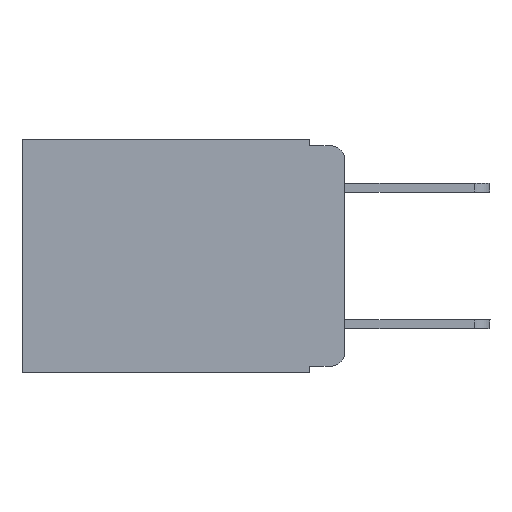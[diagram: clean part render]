
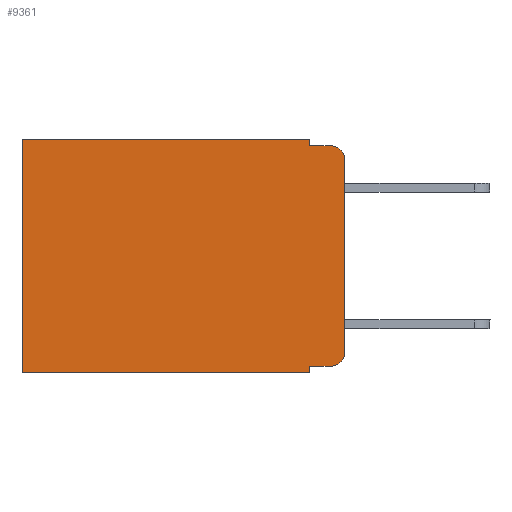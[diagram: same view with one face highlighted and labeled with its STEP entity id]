
A CAD part, left-side view. The second image highlights one B-rep face of the part: STEP entity #9361.
In plain terms, the highlighted planar face has unit normal (-1, 0, 0).
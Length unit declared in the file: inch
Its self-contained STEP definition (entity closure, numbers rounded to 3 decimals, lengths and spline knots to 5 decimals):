
#227 = EDGE_CURVE ( 'NONE', #283, #7576, #11471, .T. ) ;
#258 = VERTEX_POINT ( 'NONE', #7522 ) ;
#283 = VERTEX_POINT ( 'NONE', #7147 ) ;
#375 = CARTESIAN_POINT ( 'NONE',  ( 0.298, 0.051, -0.333 ) ) ;
#421 = EDGE_CURVE ( 'NONE', #11881, #6773, #3278, .T. ) ;
#482 = LINE ( 'NONE', #7294, #11235 ) ;
#676 = VECTOR ( 'NONE', #5127, 39.37008 ) ;
#820 = CARTESIAN_POINT ( 'NONE',  ( 0.298, 0., -0.03 ) ) ;
#1162 = CARTESIAN_POINT ( 'NONE',  ( 0.298, 0., 0. ) ) ;
#1236 = ORIENTED_EDGE ( 'NONE', *, *, #6168, .F. ) ;
#1543 = EDGE_CURVE ( 'NONE', #7630, #258, #12568, .T. ) ;
#1599 = DIRECTION ( 'NONE',  ( -1., 0., 0. ) ) ;
#1777 = CARTESIAN_POINT ( 'NONE',  ( 0.298, 0.051, 0. ) ) ;
#1807 = DIRECTION ( 'NONE',  ( -1., 0., 0. ) ) ;
#2048 = CARTESIAN_POINT ( 'NONE',  ( 0.298, 0.051, 0. ) ) ;
#2175 = FACE_OUTER_BOUND ( 'NONE', #10847, .T. ) ;
#2257 = ORIENTED_EDGE ( 'NONE', *, *, #9995, .T. ) ;
#2835 = CARTESIAN_POINT ( 'NONE',  ( 0.298, 0.473, 0. ) ) ;
#3069 = ORIENTED_EDGE ( 'NONE', *, *, #421, .T. ) ;
#3278 = LINE ( 'NONE', #2835, #5050 ) ;
#3496 = DIRECTION ( 'NONE',  ( 0., -1., 0. ) ) ;
#3521 = CARTESIAN_POINT ( 'NONE',  ( 0.298, 0., 0. ) ) ;
#3684 = DIRECTION ( 'NONE',  ( 0., 0., -1. ) ) ;
#3788 = ORIENTED_EDGE ( 'NONE', *, *, #8992, .T. ) ;
#4166 = AXIS2_PLACEMENT_3D ( 'NONE', #6722, #1599, #8792 ) ;
#4220 = ORIENTED_EDGE ( 'NONE', *, *, #9329, .T. ) ;
#4440 = VERTEX_POINT ( 'NONE', #13296 ) ;
#4481 = CIRCLE ( 'NONE', #7129, 0.02 ) ;
#4566 = CARTESIAN_POINT ( 'NONE',  ( 0.298, 0.051, -0.333 ) ) ;
#4683 = CARTESIAN_POINT ( 'NONE',  ( 0.298, 0.051, 0. ) ) ;
#4731 = DIRECTION ( 'NONE',  ( 0., 0., -1. ) ) ;
#5050 = VECTOR ( 'NONE', #8057, 39.37008 ) ;
#5127 = DIRECTION ( 'NONE',  ( 0., -1., 0. ) ) ;
#5599 = VECTOR ( 'NONE', #5652, 39.37008 ) ;
#5652 = DIRECTION ( 'NONE',  ( 0., 1., 0. ) ) ;
#5732 = EDGE_CURVE ( 'NONE', #7428, #11795, #11830, .T. ) ;
#6144 = VECTOR ( 'NONE', #3496, 39.37008 ) ;
#6168 = EDGE_CURVE ( 'NONE', #4440, #6773, #482, .T. ) ;
#6326 = DIRECTION ( 'NONE',  ( 0., 1., 0. ) ) ;
#6331 = DIRECTION ( 'NONE',  ( 0., 0., -1. ) ) ;
#6357 = EDGE_CURVE ( 'NONE', #8058, #283, #6925, .T. ) ;
#6407 = ORIENTED_EDGE ( 'NONE', *, *, #1543, .T. ) ;
#6462 = VECTOR ( 'NONE', #4731, 39.37008 ) ;
#6722 = CARTESIAN_POINT ( 'NONE',  ( 0.298, 0.02, -0.313 ) ) ;
#6773 = VERTEX_POINT ( 'NONE', #9364 ) ;
#6925 = LINE ( 'NONE', #4683, #8186 ) ;
#7129 = AXIS2_PLACEMENT_3D ( 'NONE', #11010, #1807, #12092 ) ;
#7147 = CARTESIAN_POINT ( 'NONE',  ( 0.298, 0.051, -0.01 ) ) ;
#7247 = LINE ( 'NONE', #1777, #6462 ) ;
#7294 = CARTESIAN_POINT ( 'NONE',  ( 0.298, 0., -0.343 ) ) ;
#7428 = VERTEX_POINT ( 'NONE', #820 ) ;
#7522 = CARTESIAN_POINT ( 'NONE',  ( 0.298, 0.02, -0.333 ) ) ;
#7576 = VERTEX_POINT ( 'NONE', #12349 ) ;
#7630 = VERTEX_POINT ( 'NONE', #4566 ) ;
#7655 = LINE ( 'NONE', #1162, #5599 ) ;
#8057 = DIRECTION ( 'NONE',  ( 0., 0., -1. ) ) ;
#8058 = VERTEX_POINT ( 'NONE', #2048 ) ;
#8186 = VECTOR ( 'NONE', #3684, 39.37008 ) ;
#8372 = ORIENTED_EDGE ( 'NONE', *, *, #6357, .F. ) ;
#8576 = CARTESIAN_POINT ( 'NONE',  ( 0.298, 0.473, 0. ) ) ;
#8736 = DIRECTION ( 'NONE',  ( 0., 0., -1. ) ) ;
#8792 = DIRECTION ( 'NONE',  ( 0., 0., -1. ) ) ;
#8872 = AXIS2_PLACEMENT_3D ( 'NONE', #3521, #11701, #8736 ) ;
#8992 = EDGE_CURVE ( 'NONE', #7428, #7576, #4481, .T. ) ;
#9329 = EDGE_CURVE ( 'NONE', #8058, #11881, #7655, .T. ) ;
#9361 = ADVANCED_FACE ( 'NONE', ( #2175 ), #9617, .F. ) ;
#9364 = CARTESIAN_POINT ( 'NONE',  ( 0.298, 0.473, -0.343 ) ) ;
#9617 = PLANE ( 'NONE',  #8872 ) ;
#9708 = ORIENTED_EDGE ( 'NONE', *, *, #227, .F. ) ;
#9995 = EDGE_CURVE ( 'NONE', #258, #11795, #12284, .T. ) ;
#10327 = CARTESIAN_POINT ( 'NONE',  ( 0.298, 0., 0. ) ) ;
#10734 = CARTESIAN_POINT ( 'NONE',  ( 0.298, 0., -0.313 ) ) ;
#10847 = EDGE_LOOP ( 'NONE', ( #11048, #3788, #9708, #8372, #4220, #3069, #1236, #10872, #6407, #2257 ) ) ;
#10872 = ORIENTED_EDGE ( 'NONE', *, *, #12462, .F. ) ;
#10904 = CARTESIAN_POINT ( 'NONE',  ( 0.298, 0.051, -0.01 ) ) ;
#11010 = CARTESIAN_POINT ( 'NONE',  ( 0.298, 0.02, -0.03 ) ) ;
#11048 = ORIENTED_EDGE ( 'NONE', *, *, #5732, .F. ) ;
#11235 = VECTOR ( 'NONE', #6326, 39.37008 ) ;
#11471 = LINE ( 'NONE', #10904, #676 ) ;
#11701 = DIRECTION ( 'NONE',  ( 1., 0., 0. ) ) ;
#11795 = VERTEX_POINT ( 'NONE', #10734 ) ;
#11830 = LINE ( 'NONE', #10327, #12432 ) ;
#11881 = VERTEX_POINT ( 'NONE', #8576 ) ;
#12092 = DIRECTION ( 'NONE',  ( 0., 0., -1. ) ) ;
#12284 = CIRCLE ( 'NONE', #4166, 0.02 ) ;
#12349 = CARTESIAN_POINT ( 'NONE',  ( 0.298, 0.02, -0.01 ) ) ;
#12432 = VECTOR ( 'NONE', #6331, 39.37008 ) ;
#12462 = EDGE_CURVE ( 'NONE', #7630, #4440, #7247, .T. ) ;
#12568 = LINE ( 'NONE', #375, #6144 ) ;
#13296 = CARTESIAN_POINT ( 'NONE',  ( 0.298, 0.051, -0.343 ) ) ;
